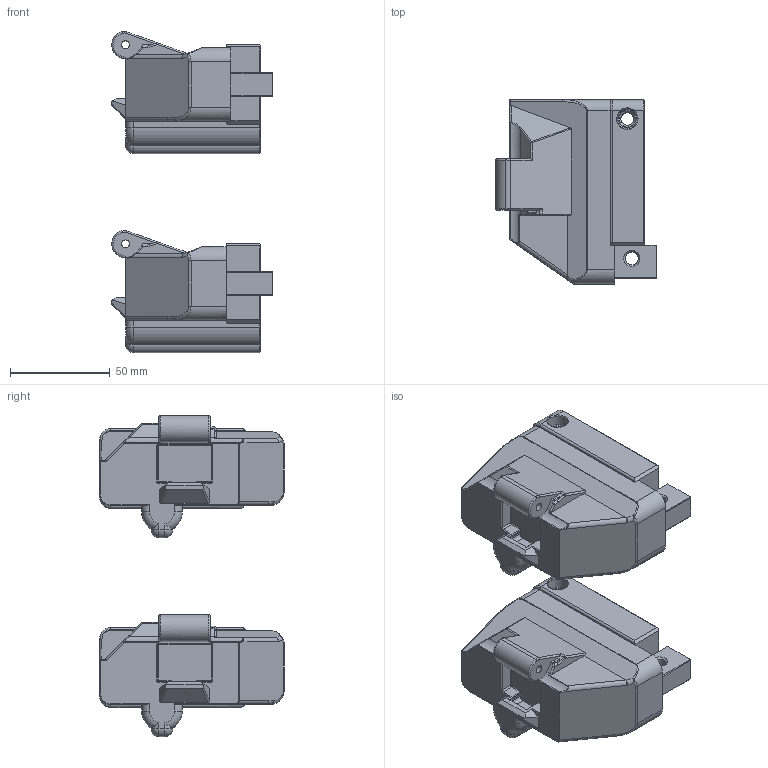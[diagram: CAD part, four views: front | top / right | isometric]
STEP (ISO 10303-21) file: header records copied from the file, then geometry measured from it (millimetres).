
FILE_DESCRIPTION(/* description */ (''),/* implementation_level */ '2;1');
FILE_NAME(/* name */ 'V2 and V3 Hinged Endcap.stp',/* time_stamp */ '2021-08-06T01:08:14+02:00',/* author */ (''),/* organization */ (''),/* preprocessor_version */ 'ST-DEVELOPER v15.2',/* originating_system */ 'Autodesk Translator Framework v2.0.0.5431',/* authorisation */ '');
FILE_SCHEMA (('AUTOMOTIVE_DESIGN { 1 0 10303 214 3 1 1 }'));
Length unit declared in the file: centimetre
Products named in the file (1): V2 and V3 Hinged Endcap
Bounding box: 80.79 x 92.64 x 161.4 mm (x, y, z)
Volume: 384301 mm3; surface area: 66318.4 mm2
Topology: 2 solids, 2 shells, 538 faces, 1363 edges, 834 vertices
Faces by surface type: plane 210, cylinder 179, bspline 54, torus 46, cone 39, sphere 10
Full cylindrical faces by diameter (mm): 4 x3, 6.5 x6, 10 x4, 13 x2, 27.4 x2
Entity records: 18499 total; most frequent: CARTESIAN_POINT 5799, DIRECTION 2649, ORIENTED_EDGE 2620, EDGE_CURVE 1310, AXIS2_PLACEMENT_3D 958, VERTEX_POINT 821, LINE 733, VECTOR 733
